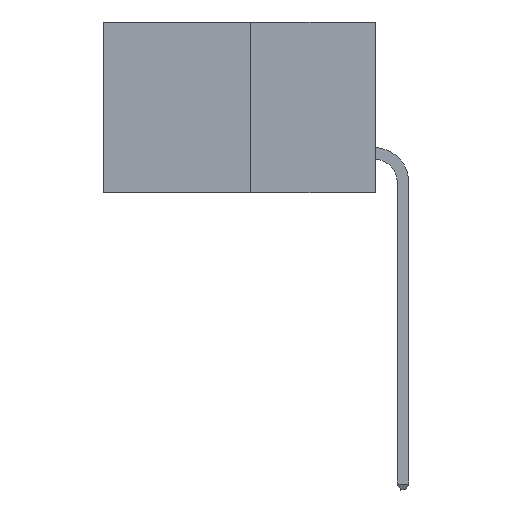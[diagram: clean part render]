
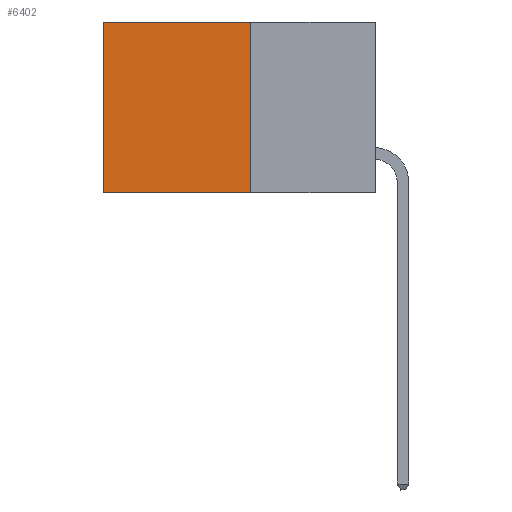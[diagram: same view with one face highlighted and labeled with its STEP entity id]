
A CAD part, left-side view. The second image highlights one B-rep face of the part: STEP entity #6402.
In plain terms, the highlighted planar face has unit normal (-1, 0, 0).
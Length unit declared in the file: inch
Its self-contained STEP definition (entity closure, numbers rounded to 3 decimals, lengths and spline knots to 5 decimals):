
#31 = EDGE_CURVE ( 'NONE', #1483, #14628, #11937, .T. ) ;
#285 = DIRECTION ( 'NONE',  ( 0., 0., -1. ) ) ;
#896 = VECTOR ( 'NONE', #5354, 39.37008 ) ;
#1483 = VERTEX_POINT ( 'NONE', #14498 ) ;
#4244 = VECTOR ( 'NONE', #10497, 39.37008 ) ;
#4867 = VECTOR ( 'NONE', #8077, 39.37008 ) ;
#5344 = VERTEX_POINT ( 'NONE', #11375 ) ;
#5354 = DIRECTION ( 'NONE',  ( 0., 1., 0. ) ) ;
#5462 = CARTESIAN_POINT ( 'NONE',  ( 0.277, 0.59, -0.37 ) ) ;
#5835 = EDGE_LOOP ( 'NONE', ( #7248, #10122, #11505, #7363 ) ) ;
#6226 = PLANE ( 'NONE',  #9796 ) ;
#6402 = ADVANCED_FACE ( 'NONE', ( #8085 ), #6226, .F. ) ;
#6860 = CARTESIAN_POINT ( 'NONE',  ( 0.277, 0.27, -0.37 ) ) ;
#6910 = EDGE_CURVE ( 'NONE', #14518, #14628, #10013, .T. ) ;
#7248 = ORIENTED_EDGE ( 'NONE', *, *, #6910, .T. ) ;
#7363 = ORIENTED_EDGE ( 'NONE', *, *, #12521, .T. ) ;
#7416 = DIRECTION ( 'NONE',  ( 1., 0., 0. ) ) ;
#7608 = CARTESIAN_POINT ( 'NONE',  ( 0.277, 0.59, 0. ) ) ;
#8077 = DIRECTION ( 'NONE',  ( 0., 0., -1. ) ) ;
#8085 = FACE_OUTER_BOUND ( 'NONE', #5835, .T. ) ;
#8837 = CARTESIAN_POINT ( 'NONE',  ( 0.277, 0.27, 0. ) ) ;
#9402 = CARTESIAN_POINT ( 'NONE',  ( 0.277, 0.59, -0.37 ) ) ;
#9796 = AXIS2_PLACEMENT_3D ( 'NONE', #13958, #7416, #285 ) ;
#9898 = LINE ( 'NONE', #8837, #896 ) ;
#10013 = LINE ( 'NONE', #9402, #4244 ) ;
#10122 = ORIENTED_EDGE ( 'NONE', *, *, #31, .F. ) ;
#10276 = EDGE_CURVE ( 'NONE', #5344, #1483, #13746, .T. ) ;
#10497 = DIRECTION ( 'NONE',  ( 0., 0., -1. ) ) ;
#11375 = CARTESIAN_POINT ( 'NONE',  ( 0.277, 0.27, 0. ) ) ;
#11505 = ORIENTED_EDGE ( 'NONE', *, *, #10276, .F. ) ;
#11613 = VECTOR ( 'NONE', #11778, 39.37008 ) ;
#11778 = DIRECTION ( 'NONE',  ( 0., 1., 0. ) ) ;
#11873 = CARTESIAN_POINT ( 'NONE',  ( 0.277, 0.27, -0.37 ) ) ;
#11937 = LINE ( 'NONE', #11873, #11613 ) ;
#12521 = EDGE_CURVE ( 'NONE', #5344, #14518, #9898, .T. ) ;
#13746 = LINE ( 'NONE', #6860, #4867 ) ;
#13958 = CARTESIAN_POINT ( 'NONE',  ( 0.277, 0.27, -0.37 ) ) ;
#14498 = CARTESIAN_POINT ( 'NONE',  ( 0.277, 0.27, -0.37 ) ) ;
#14518 = VERTEX_POINT ( 'NONE', #7608 ) ;
#14628 = VERTEX_POINT ( 'NONE', #5462 ) ;
